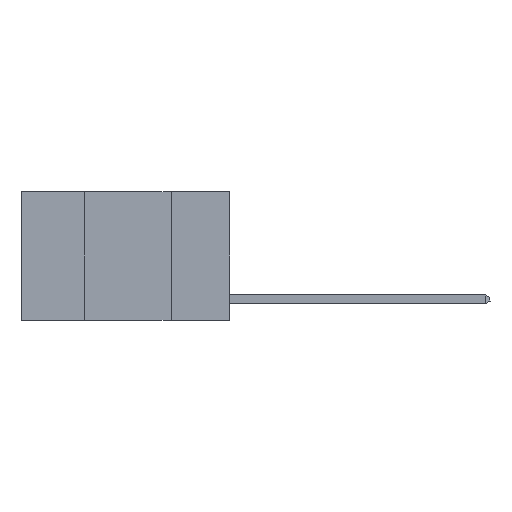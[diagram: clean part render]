
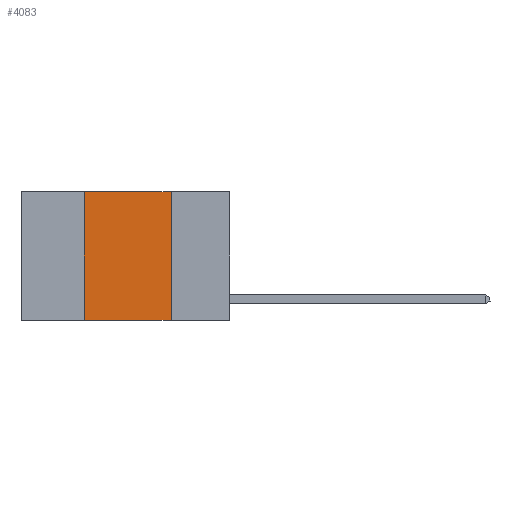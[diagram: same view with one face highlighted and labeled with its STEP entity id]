
A CAD part, left-side view. The second image highlights one B-rep face of the part: STEP entity #4083.
In plain terms, the highlighted planar face has unit normal (-1, 0, 0).
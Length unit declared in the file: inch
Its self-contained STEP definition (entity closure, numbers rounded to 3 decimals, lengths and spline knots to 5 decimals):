
#631 = DIRECTION ( 'NONE',  ( 0., 0., -1. ) ) ;
#1345 = ORIENTED_EDGE ( 'NONE', *, *, #3480, .T. ) ;
#3203 = CARTESIAN_POINT ( 'NONE',  ( 0., 0.17, 0. ) ) ;
#3480 = EDGE_CURVE ( 'NONE', #12113, #7218, #13695, .T. ) ;
#3684 = EDGE_LOOP ( 'NONE', ( #11096, #11477, #13638, #1345 ) ) ;
#3780 = VERTEX_POINT ( 'NONE', #3203 ) ;
#3918 = CARTESIAN_POINT ( 'NONE',  ( 0., 0.6, -0.37 ) ) ;
#4083 = ADVANCED_FACE ( 'NONE', ( #17189 ), #7060, .F. ) ;
#4191 = DIRECTION ( 'NONE',  ( 1., 0., 0. ) ) ;
#5377 = AXIS2_PLACEMENT_3D ( 'NONE', #14337, #4191, #11602 ) ;
#6168 = DIRECTION ( 'NONE',  ( 0., 0., 1. ) ) ;
#7060 = PLANE ( 'NONE',  #5377 ) ;
#7218 = VERTEX_POINT ( 'NONE', #9372 ) ;
#7922 = DIRECTION ( 'NONE',  ( 0., -1., 0. ) ) ;
#8053 = VERTEX_POINT ( 'NONE', #18811 ) ;
#8849 = LINE ( 'NONE', #11775, #11133 ) ;
#9067 = DIRECTION ( 'NONE',  ( 0., -1., 0. ) ) ;
#9273 = CARTESIAN_POINT ( 'NONE',  ( 0., 0.17, 0. ) ) ;
#9372 = CARTESIAN_POINT ( 'NONE',  ( 0., 0.17, -0.37 ) ) ;
#9567 = VECTOR ( 'NONE', #631, 39.37008 ) ;
#10313 = EDGE_CURVE ( 'NONE', #8053, #3780, #13510, .T. ) ;
#11096 = ORIENTED_EDGE ( 'NONE', *, *, #12512, .F. ) ;
#11133 = VECTOR ( 'NONE', #6168, 39.37008 ) ;
#11477 = ORIENTED_EDGE ( 'NONE', *, *, #10313, .F. ) ;
#11602 = DIRECTION ( 'NONE',  ( 0., 0., -1. ) ) ;
#11775 = CARTESIAN_POINT ( 'NONE',  ( 0., 0.42, 0. ) ) ;
#12053 = VECTOR ( 'NONE', #9067, 39.37008 ) ;
#12113 = VERTEX_POINT ( 'NONE', #16577 ) ;
#12512 = EDGE_CURVE ( 'NONE', #3780, #7218, #15126, .T. ) ;
#13510 = LINE ( 'NONE', #14835, #12053 ) ;
#13638 = ORIENTED_EDGE ( 'NONE', *, *, #13853, .F. ) ;
#13695 = LINE ( 'NONE', #3918, #14062 ) ;
#13853 = EDGE_CURVE ( 'NONE', #12113, #8053, #8849, .T. ) ;
#14062 = VECTOR ( 'NONE', #7922, 39.37008 ) ;
#14337 = CARTESIAN_POINT ( 'NONE',  ( 0., 0.6, 0. ) ) ;
#14835 = CARTESIAN_POINT ( 'NONE',  ( 0., 0.6, 0. ) ) ;
#15126 = LINE ( 'NONE', #9273, #9567 ) ;
#16577 = CARTESIAN_POINT ( 'NONE',  ( 0., 0.42, -0.37 ) ) ;
#17189 = FACE_OUTER_BOUND ( 'NONE', #3684, .T. ) ;
#18811 = CARTESIAN_POINT ( 'NONE',  ( 0., 0.42, 0. ) ) ;
